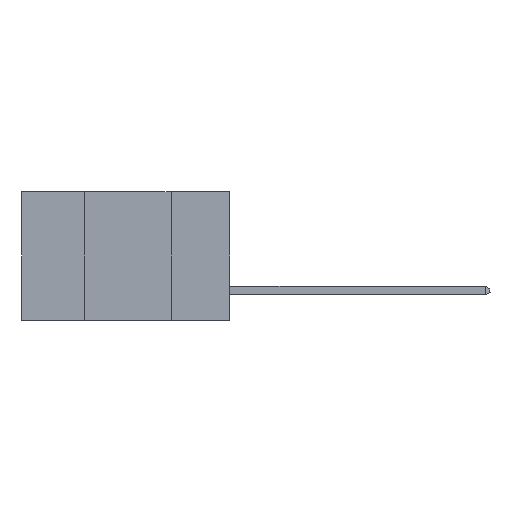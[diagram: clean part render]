
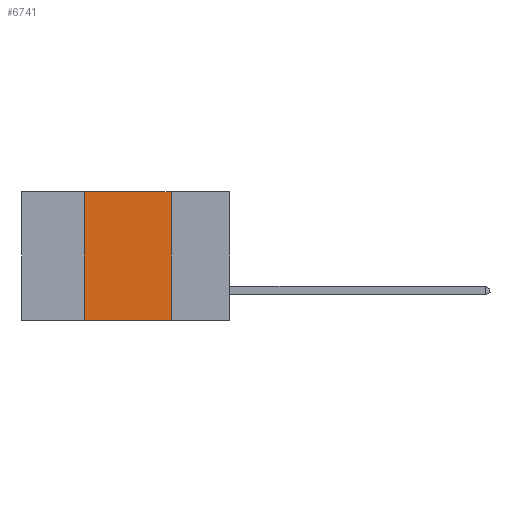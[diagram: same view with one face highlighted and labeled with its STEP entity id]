
A CAD part, left-side view. The second image highlights one B-rep face of the part: STEP entity #6741.
In plain terms, the highlighted planar face has unit normal (-1, 0, 0).
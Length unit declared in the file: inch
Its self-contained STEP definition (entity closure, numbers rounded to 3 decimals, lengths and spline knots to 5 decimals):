
#69 = CARTESIAN_POINT ( 'NONE',  ( 0., 0.42, 0. ) ) ;
#2206 = EDGE_CURVE ( 'NONE', #9956, #25361, #17596, .T. ) ;
#5009 = ORIENTED_EDGE ( 'NONE', *, *, #9698, .F. ) ;
#5108 = DIRECTION ( 'NONE',  ( 0., -1., 0. ) ) ;
#5304 = VERTEX_POINT ( 'NONE', #17427 ) ;
#6573 = ORIENTED_EDGE ( 'NONE', *, *, #17789, .T. ) ;
#6741 = ADVANCED_FACE ( 'NONE', ( #22635 ), #23028, .F. ) ;
#7090 = CARTESIAN_POINT ( 'NONE',  ( 0., 0.6, 0. ) ) ;
#8929 = ORIENTED_EDGE ( 'NONE', *, *, #23392, .F. ) ;
#9698 = EDGE_CURVE ( 'NONE', #5304, #9956, #17172, .T. ) ;
#9956 = VERTEX_POINT ( 'NONE', #69 ) ;
#11936 = VERTEX_POINT ( 'NONE', #16498 ) ;
#12849 = LINE ( 'NONE', #19774, #17487 ) ;
#13143 = DIRECTION ( 'NONE',  ( 0., 0., -1. ) ) ;
#13321 = ORIENTED_EDGE ( 'NONE', *, *, #2206, .F. ) ;
#14885 = CARTESIAN_POINT ( 'NONE',  ( 0., 0.17, 0. ) ) ;
#15738 = CARTESIAN_POINT ( 'NONE',  ( 0., 0.42, 0. ) ) ;
#16006 = EDGE_LOOP ( 'NONE', ( #8929, #13321, #5009, #6573 ) ) ;
#16281 = VECTOR ( 'NONE', #21092, 39.37008 ) ;
#16498 = CARTESIAN_POINT ( 'NONE',  ( 0., 0.17, -0.37 ) ) ;
#17018 = CARTESIAN_POINT ( 'NONE',  ( 0., 0.6, 0. ) ) ;
#17172 = LINE ( 'NONE', #15738, #21227 ) ;
#17264 = CARTESIAN_POINT ( 'NONE',  ( 0., 0.17, 0. ) ) ;
#17427 = CARTESIAN_POINT ( 'NONE',  ( 0., 0.42, -0.37 ) ) ;
#17487 = VECTOR ( 'NONE', #23511, 39.37008 ) ;
#17596 = LINE ( 'NONE', #17018, #21650 ) ;
#17789 = EDGE_CURVE ( 'NONE', #5304, #11936, #12849, .T. ) ;
#18746 = LINE ( 'NONE', #14885, #16281 ) ;
#19774 = CARTESIAN_POINT ( 'NONE',  ( 0., 0.6, -0.37 ) ) ;
#21092 = DIRECTION ( 'NONE',  ( 0., 0., -1. ) ) ;
#21227 = VECTOR ( 'NONE', #21634, 39.37008 ) ;
#21634 = DIRECTION ( 'NONE',  ( 0., 0., 1. ) ) ;
#21650 = VECTOR ( 'NONE', #5108, 39.37008 ) ;
#22635 = FACE_OUTER_BOUND ( 'NONE', #16006, .T. ) ;
#23028 = PLANE ( 'NONE',  #25050 ) ;
#23392 = EDGE_CURVE ( 'NONE', #25361, #11936, #18746, .T. ) ;
#23511 = DIRECTION ( 'NONE',  ( 0., -1., 0. ) ) ;
#25012 = DIRECTION ( 'NONE',  ( 1., 0., 0. ) ) ;
#25050 = AXIS2_PLACEMENT_3D ( 'NONE', #7090, #25012, #13143 ) ;
#25361 = VERTEX_POINT ( 'NONE', #17264 ) ;
